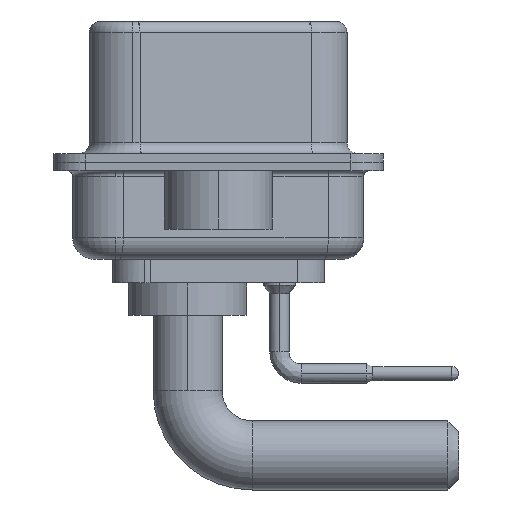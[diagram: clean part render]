
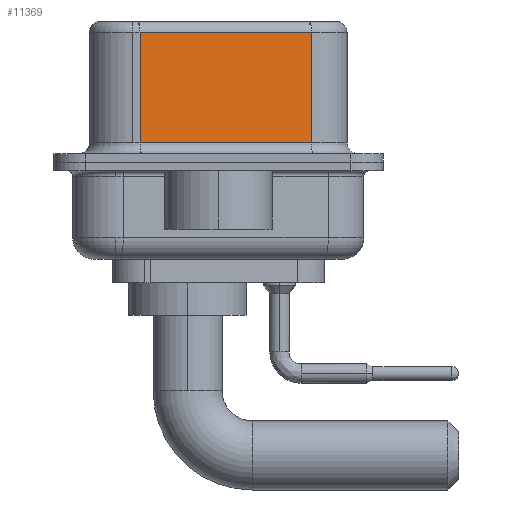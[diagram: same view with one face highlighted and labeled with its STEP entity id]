
A CAD part, left-side view. The second image highlights one B-rep face of the part: STEP entity #11369.
In plain terms, the highlighted planar face has unit normal (-0.985, -0.174, 0).
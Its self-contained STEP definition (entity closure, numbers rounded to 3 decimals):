
#149 = DIRECTION ( 'NONE',  ( 0., 0., -1. ) ) ;
#152 = EDGE_CURVE ( 'NONE', #1789, #530, #8158, .T. ) ;
#380 = ORIENTED_EDGE ( 'NONE', *, *, #20858, .T. ) ;
#530 = VERTEX_POINT ( 'NONE', #13445 ) ;
#1117 = AXIS2_PLACEMENT_3D ( 'NONE', #11811, #22703, #22942 ) ;
#1650 = VECTOR ( 'NONE', #22541, 1000. ) ;
#1737 = CARTESIAN_POINT ( 'NONE',  ( 3.73, 3.628, 6.52 ) ) ;
#1789 = VERTEX_POINT ( 'NONE', #9730 ) ;
#2459 = VERTEX_POINT ( 'NONE', #9176 ) ;
#2575 = LINE ( 'NONE', #22410, #23468 ) ;
#4262 = DIRECTION ( 'NONE',  ( 0.174, -0.985, 0. ) ) ;
#4433 = FACE_OUTER_BOUND ( 'NONE', #5287, .T. ) ;
#4488 = ORIENTED_EDGE ( 'NONE', *, *, #8001, .F. ) ;
#5245 = LINE ( 'NONE', #1737, #5968 ) ;
#5287 = EDGE_LOOP ( 'NONE', ( #4488, #15467, #14465, #380 ) ) ;
#5724 = DIRECTION ( 'NONE',  ( 0., 0., -1. ) ) ;
#5968 = VECTOR ( 'NONE', #149, 1000. ) ;
#6101 = CARTESIAN_POINT ( 'NONE',  ( 5.132, -4.322, 6.02 ) ) ;
#7722 = CARTESIAN_POINT ( 'NONE',  ( 3.73, 3.628, 0.9 ) ) ;
#8001 = EDGE_CURVE ( 'NONE', #1789, #2459, #2575, .T. ) ;
#8158 = LINE ( 'NONE', #6101, #1650 ) ;
#9176 = CARTESIAN_POINT ( 'NONE',  ( 5.132, -4.322, 0.9 ) ) ;
#9730 = CARTESIAN_POINT ( 'NONE',  ( 5.132, -4.322, 6.02 ) ) ;
#11369 = ADVANCED_FACE ( 'NONE', ( #4433 ), #15329, .F. ) ;
#11755 = CARTESIAN_POINT ( 'NONE',  ( 5.132, -4.322, 0.9 ) ) ;
#11811 = CARTESIAN_POINT ( 'NONE',  ( 5.132, -4.322, 6.52 ) ) ;
#12792 = VECTOR ( 'NONE', #4262, 1000. ) ;
#13445 = CARTESIAN_POINT ( 'NONE',  ( 3.73, 3.628, 6.02 ) ) ;
#13934 = LINE ( 'NONE', #11755, #12792 ) ;
#14465 = ORIENTED_EDGE ( 'NONE', *, *, #23553, .T. ) ;
#15329 = PLANE ( 'NONE',  #1117 ) ;
#15467 = ORIENTED_EDGE ( 'NONE', *, *, #152, .T. ) ;
#20858 = EDGE_CURVE ( 'NONE', #22715, #2459, #13934, .T. ) ;
#22410 = CARTESIAN_POINT ( 'NONE',  ( 5.132, -4.322, 6.52 ) ) ;
#22541 = DIRECTION ( 'NONE',  ( -0.174, 0.985, 0. ) ) ;
#22703 = DIRECTION ( 'NONE',  ( 0.985, 0.174, 0. ) ) ;
#22715 = VERTEX_POINT ( 'NONE', #7722 ) ;
#22942 = DIRECTION ( 'NONE',  ( -0.174, 0.985, 0. ) ) ;
#23468 = VECTOR ( 'NONE', #5724, 1000. ) ;
#23553 = EDGE_CURVE ( 'NONE', #530, #22715, #5245, .T. ) ;
